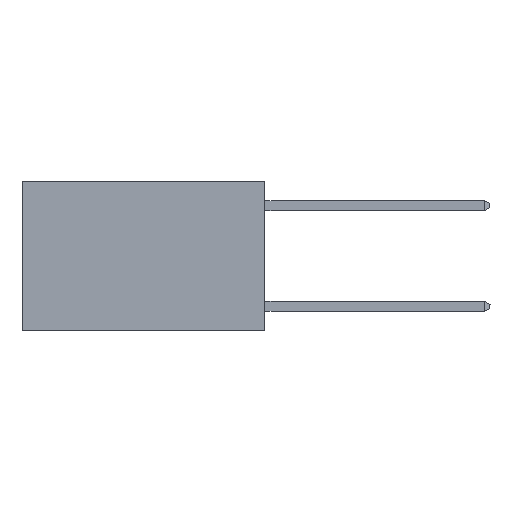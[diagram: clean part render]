
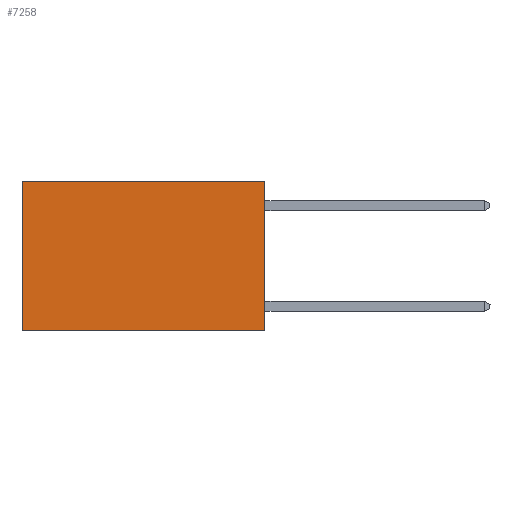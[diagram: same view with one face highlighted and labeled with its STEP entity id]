
A CAD part, left-side view. The second image highlights one B-rep face of the part: STEP entity #7258.
In plain terms, the highlighted planar face has unit normal (-1, 0, 0).
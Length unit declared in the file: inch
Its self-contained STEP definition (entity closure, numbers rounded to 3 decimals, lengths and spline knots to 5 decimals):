
#143 = VECTOR ( 'NONE', #6969, 39.37008 ) ;
#270 = ORIENTED_EDGE ( 'NONE', *, *, #855, .F. ) ;
#533 = ORIENTED_EDGE ( 'NONE', *, *, #3054, .F. ) ;
#540 = AXIS2_PLACEMENT_3D ( 'NONE', #2124, #3014, #8816 ) ;
#855 = EDGE_CURVE ( 'NONE', #10121, #2437, #1133, .T. ) ;
#871 = LINE ( 'NONE', #1016, #5209 ) ;
#1016 = CARTESIAN_POINT ( 'NONE',  ( 0.2625, 0.6, 0. ) ) ;
#1133 = LINE ( 'NONE', #5421, #143 ) ;
#1189 = PLANE ( 'NONE',  #540 ) ;
#1220 = ORIENTED_EDGE ( 'NONE', *, *, #3138, .T. ) ;
#1303 = DIRECTION ( 'NONE',  ( 0., 0., -1. ) ) ;
#1904 = CARTESIAN_POINT ( 'NONE',  ( 0.2625, 0., -0.37 ) ) ;
#2124 = CARTESIAN_POINT ( 'NONE',  ( 0.2625, 0., 0. ) ) ;
#2437 = VERTEX_POINT ( 'NONE', #9832 ) ;
#2499 = EDGE_LOOP ( 'NONE', ( #1220, #533, #270, #8615 ) ) ;
#3014 = DIRECTION ( 'NONE',  ( 1., 0., 0. ) ) ;
#3054 = EDGE_CURVE ( 'NONE', #2437, #10933, #5729, .T. ) ;
#3138 = EDGE_CURVE ( 'NONE', #3176, #10933, #871, .T. ) ;
#3176 = VERTEX_POINT ( 'NONE', #6269 ) ;
#3595 = LINE ( 'NONE', #7811, #7754 ) ;
#5011 = FACE_OUTER_BOUND ( 'NONE', #2499, .T. ) ;
#5209 = VECTOR ( 'NONE', #1303, 39.37008 ) ;
#5421 = CARTESIAN_POINT ( 'NONE',  ( 0.2625, 0., 0. ) ) ;
#5579 = DIRECTION ( 'NONE',  ( 0., 1., 0. ) ) ;
#5729 = LINE ( 'NONE', #1904, #7711 ) ;
#6269 = CARTESIAN_POINT ( 'NONE',  ( 0.2625, 0.6, 0. ) ) ;
#6350 = CARTESIAN_POINT ( 'NONE',  ( 0.2625, 0.6, -0.37 ) ) ;
#6969 = DIRECTION ( 'NONE',  ( 0., 0., -1. ) ) ;
#7258 = ADVANCED_FACE ( 'NONE', ( #5011 ), #1189, .F. ) ;
#7542 = EDGE_CURVE ( 'NONE', #10121, #3176, #3595, .T. ) ;
#7711 = VECTOR ( 'NONE', #5579, 39.37008 ) ;
#7754 = VECTOR ( 'NONE', #8588, 39.37008 ) ;
#7811 = CARTESIAN_POINT ( 'NONE',  ( 0.2625, 0., 0. ) ) ;
#8588 = DIRECTION ( 'NONE',  ( 0., 1., 0. ) ) ;
#8615 = ORIENTED_EDGE ( 'NONE', *, *, #7542, .T. ) ;
#8816 = DIRECTION ( 'NONE',  ( 0., 0., -1. ) ) ;
#8938 = CARTESIAN_POINT ( 'NONE',  ( 0.2625, 0., 0. ) ) ;
#9832 = CARTESIAN_POINT ( 'NONE',  ( 0.2625, 0., -0.37 ) ) ;
#10121 = VERTEX_POINT ( 'NONE', #8938 ) ;
#10933 = VERTEX_POINT ( 'NONE', #6350 ) ;
